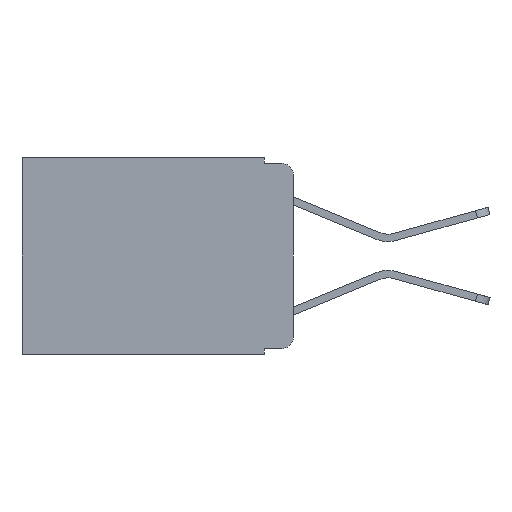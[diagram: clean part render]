
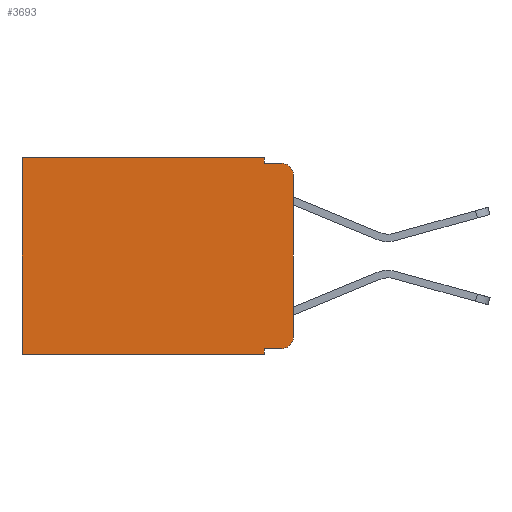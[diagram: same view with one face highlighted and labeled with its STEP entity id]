
A CAD part, left-side view. The second image highlights one B-rep face of the part: STEP entity #3693.
In plain terms, the highlighted planar face has unit normal (-1, 0, 0).
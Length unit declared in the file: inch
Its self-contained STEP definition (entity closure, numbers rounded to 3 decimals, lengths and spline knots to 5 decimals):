
#40 = VERTEX_POINT ( 'NONE', #8834 ) ;
#107 = CARTESIAN_POINT ( 'NONE',  ( 0.298, 0.051, -0.343 ) ) ;
#192 = EDGE_CURVE ( 'NONE', #4315, #4771, #1164, .T. ) ;
#200 = ORIENTED_EDGE ( 'NONE', *, *, #7682, .F. ) ;
#372 = EDGE_CURVE ( 'NONE', #40, #5689, #8657, .T. ) ;
#402 = AXIS2_PLACEMENT_3D ( 'NONE', #5233, #3686, #4482 ) ;
#713 = ORIENTED_EDGE ( 'NONE', *, *, #10301, .T. ) ;
#721 = CARTESIAN_POINT ( 'NONE',  ( 0.298, 0.051, 0. ) ) ;
#973 = LINE ( 'NONE', #6085, #5847 ) ;
#1164 = LINE ( 'NONE', #7264, #4553 ) ;
#1218 = FACE_OUTER_BOUND ( 'NONE', #6941, .T. ) ;
#1299 = DIRECTION ( 'NONE',  ( 0., -1., 0. ) ) ;
#1498 = VECTOR ( 'NONE', #1612, 39.37008 ) ;
#1612 = DIRECTION ( 'NONE',  ( 0., 0., -1. ) ) ;
#1691 = CARTESIAN_POINT ( 'NONE',  ( 0.298, 0.473, -0.343 ) ) ;
#2002 = CARTESIAN_POINT ( 'NONE',  ( 0.298, 0.051, -0.333 ) ) ;
#2012 = VECTOR ( 'NONE', #2323, 39.37008 ) ;
#2062 = CARTESIAN_POINT ( 'NONE',  ( 0.298, 0.473, 0. ) ) ;
#2103 = LINE ( 'NONE', #2062, #7741 ) ;
#2204 = ORIENTED_EDGE ( 'NONE', *, *, #8548, .T. ) ;
#2265 = CARTESIAN_POINT ( 'NONE',  ( 0.298, 0.051, 0. ) ) ;
#2323 = DIRECTION ( 'NONE',  ( 0., 0., -1. ) ) ;
#2404 = CARTESIAN_POINT ( 'NONE',  ( 0.298, 0., 0. ) ) ;
#2483 = ORIENTED_EDGE ( 'NONE', *, *, #5719, .F. ) ;
#2542 = AXIS2_PLACEMENT_3D ( 'NONE', #8094, #7313, #8130 ) ;
#2611 = CARTESIAN_POINT ( 'NONE',  ( 0.298, 0.02, -0.01 ) ) ;
#2881 = DIRECTION ( 'NONE',  ( 0., 0., -1. ) ) ;
#2951 = VERTEX_POINT ( 'NONE', #3039 ) ;
#2953 = ORIENTED_EDGE ( 'NONE', *, *, #192, .F. ) ;
#3039 = CARTESIAN_POINT ( 'NONE',  ( 0.298, 0.051, -0.333 ) ) ;
#3545 = ORIENTED_EDGE ( 'NONE', *, *, #372, .F. ) ;
#3686 = DIRECTION ( 'NONE',  ( -1., 0., 0. ) ) ;
#3693 = ADVANCED_FACE ( 'NONE', ( #1218 ), #9986, .F. ) ;
#4035 = VERTEX_POINT ( 'NONE', #4328 ) ;
#4252 = CARTESIAN_POINT ( 'NONE',  ( 0.298, 0.051, -0.01 ) ) ;
#4315 = VERTEX_POINT ( 'NONE', #107 ) ;
#4328 = CARTESIAN_POINT ( 'NONE',  ( 0.298, 0.473, 0. ) ) ;
#4468 = DIRECTION ( 'NONE',  ( 0., 0., -1. ) ) ;
#4482 = DIRECTION ( 'NONE',  ( 0., 0., -1. ) ) ;
#4553 = VECTOR ( 'NONE', #8075, 39.37008 ) ;
#4771 = VERTEX_POINT ( 'NONE', #1691 ) ;
#4804 = ORIENTED_EDGE ( 'NONE', *, *, #8690, .T. ) ;
#4844 = ORIENTED_EDGE ( 'NONE', *, *, #8987, .F. ) ;
#5233 = CARTESIAN_POINT ( 'NONE',  ( 0.298, 0.02, -0.03 ) ) ;
#5236 = CARTESIAN_POINT ( 'NONE',  ( 0.298, 0.02, -0.333 ) ) ;
#5237 = CIRCLE ( 'NONE', #2542, 0.02 ) ;
#5612 = CARTESIAN_POINT ( 'NONE',  ( 0.298, 0., 0. ) ) ;
#5689 = VERTEX_POINT ( 'NONE', #6629 ) ;
#5719 = EDGE_CURVE ( 'NONE', #8782, #8536, #6513, .T. ) ;
#5720 = AXIS2_PLACEMENT_3D ( 'NONE', #6066, #6100, #4468 ) ;
#5847 = VECTOR ( 'NONE', #1299, 39.37008 ) ;
#6066 = CARTESIAN_POINT ( 'NONE',  ( 0.298, 0., 0. ) ) ;
#6085 = CARTESIAN_POINT ( 'NONE',  ( 0.298, 0.051, -0.01 ) ) ;
#6100 = DIRECTION ( 'NONE',  ( 1., 0., 0. ) ) ;
#6328 = CARTESIAN_POINT ( 'NONE',  ( 0.298, 0.051, 0. ) ) ;
#6513 = LINE ( 'NONE', #721, #2012 ) ;
#6629 = CARTESIAN_POINT ( 'NONE',  ( 0.298, 0., -0.313 ) ) ;
#6816 = LINE ( 'NONE', #2002, #9965 ) ;
#6941 = EDGE_LOOP ( 'NONE', ( #3545, #8344, #4844, #2483, #7700, #4804, #2953, #200, #713, #2204 ) ) ;
#7264 = CARTESIAN_POINT ( 'NONE',  ( 0.298, 0., -0.343 ) ) ;
#7310 = DIRECTION ( 'NONE',  ( 0., 0., -1. ) ) ;
#7313 = DIRECTION ( 'NONE',  ( -1., 0., 0. ) ) ;
#7682 = EDGE_CURVE ( 'NONE', #2951, #4315, #9514, .T. ) ;
#7700 = ORIENTED_EDGE ( 'NONE', *, *, #8353, .T. ) ;
#7741 = VECTOR ( 'NONE', #2881, 39.37008 ) ;
#8026 = DIRECTION ( 'NONE',  ( 0., 1., 0. ) ) ;
#8075 = DIRECTION ( 'NONE',  ( 0., 1., 0. ) ) ;
#8094 = CARTESIAN_POINT ( 'NONE',  ( 0.298, 0.02, -0.313 ) ) ;
#8130 = DIRECTION ( 'NONE',  ( 0., 0., -1. ) ) ;
#8155 = EDGE_CURVE ( 'NONE', #40, #9480, #8864, .T. ) ;
#8344 = ORIENTED_EDGE ( 'NONE', *, *, #8155, .T. ) ;
#8353 = EDGE_CURVE ( 'NONE', #8782, #4035, #9627, .T. ) ;
#8536 = VERTEX_POINT ( 'NONE', #4252 ) ;
#8548 = EDGE_CURVE ( 'NONE', #9141, #5689, #5237, .T. ) ;
#8657 = LINE ( 'NONE', #5612, #9792 ) ;
#8690 = EDGE_CURVE ( 'NONE', #4035, #4771, #2103, .T. ) ;
#8782 = VERTEX_POINT ( 'NONE', #2265 ) ;
#8834 = CARTESIAN_POINT ( 'NONE',  ( 0.298, 0., -0.03 ) ) ;
#8864 = CIRCLE ( 'NONE', #402, 0.02 ) ;
#8987 = EDGE_CURVE ( 'NONE', #8536, #9480, #973, .T. ) ;
#9141 = VERTEX_POINT ( 'NONE', #5236 ) ;
#9480 = VERTEX_POINT ( 'NONE', #2611 ) ;
#9514 = LINE ( 'NONE', #6328, #1498 ) ;
#9627 = LINE ( 'NONE', #2404, #10258 ) ;
#9792 = VECTOR ( 'NONE', #7310, 39.37008 ) ;
#9965 = VECTOR ( 'NONE', #9983, 39.37008 ) ;
#9983 = DIRECTION ( 'NONE',  ( 0., -1., 0. ) ) ;
#9986 = PLANE ( 'NONE',  #5720 ) ;
#10258 = VECTOR ( 'NONE', #8026, 39.37008 ) ;
#10301 = EDGE_CURVE ( 'NONE', #2951, #9141, #6816, .T. ) ;
